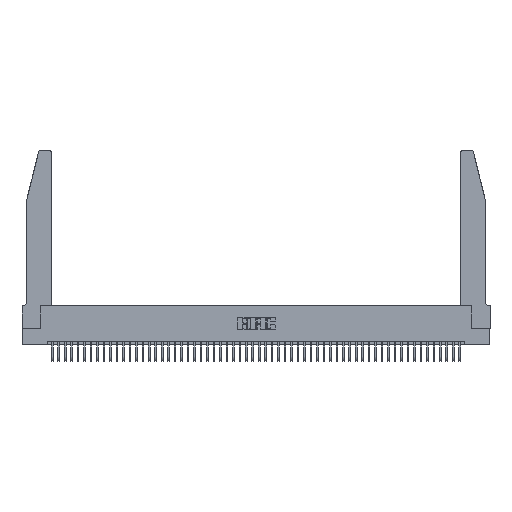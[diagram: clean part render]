
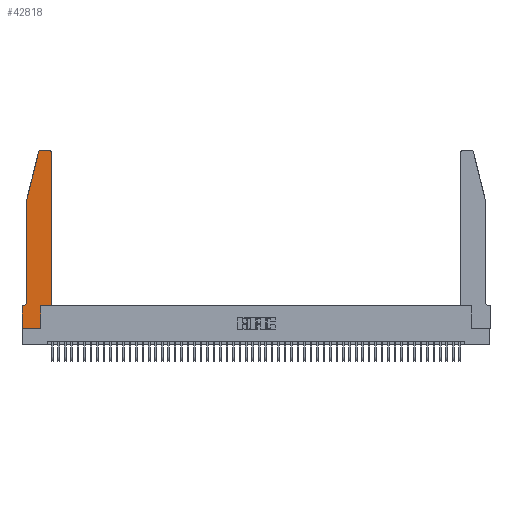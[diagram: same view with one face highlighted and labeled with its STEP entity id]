
A CAD part, top view. The second image highlights one B-rep face of the part: STEP entity #42818.
In plain terms, the highlighted planar face has unit normal (0, 0, 1).
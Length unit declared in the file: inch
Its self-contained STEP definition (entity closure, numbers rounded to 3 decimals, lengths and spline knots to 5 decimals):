
#432 = CARTESIAN_POINT ( 'NONE',  ( 0.4505, 0.35, 0.37 ) ) ;
#1032 = ORIENTED_EDGE ( 'NONE', *, *, #32963, .T. ) ;
#1326 = ORIENTED_EDGE ( 'NONE', *, *, #33201, .T. ) ;
#2645 = VERTEX_POINT ( 'NONE', #17183 ) ;
#3029 = EDGE_CURVE ( 'NONE', #3088, #14454, #19236, .T. ) ;
#3088 = VERTEX_POINT ( 'NONE', #35722 ) ;
#3173 = ORIENTED_EDGE ( 'NONE', *, *, #40153, .T. ) ;
#3395 = ORIENTED_EDGE ( 'NONE', *, *, #49207, .T. ) ;
#3697 = VERTEX_POINT ( 'NONE', #4847 ) ;
#4013 = VECTOR ( 'NONE', #29248, 39.37008 ) ;
#4138 = CARTESIAN_POINT ( 'NONE',  ( 0.4205, 2.75, 0.37 ) ) ;
#4597 = LINE ( 'NONE', #30398, #33091 ) ;
#4698 = VERTEX_POINT ( 'NONE', #19447 ) ;
#4748 = EDGE_CURVE ( 'NONE', #10122, #2645, #46123, .T. ) ;
#4847 = CARTESIAN_POINT ( 'NONE',  ( 0.0755, 2., 0.37 ) ) ;
#6041 = LINE ( 'NONE', #33193, #32089 ) ;
#6092 = DIRECTION ( 'NONE',  ( 0., -1., 0. ) ) ;
#6911 = PLANE ( 'NONE',  #46833 ) ;
#7537 = LINE ( 'NONE', #32663, #26944 ) ;
#7711 = VECTOR ( 'NONE', #12213, 39.37008 ) ;
#7830 = CARTESIAN_POINT ( 'NONE',  ( 0.2865, 0.35, 0.37 ) ) ;
#7932 = DIRECTION ( 'NONE',  ( 0., 1., 0. ) ) ;
#8380 = DIRECTION ( 'NONE',  ( 0., 0., 1. ) ) ;
#8432 = VERTEX_POINT ( 'NONE', #39535 ) ;
#8803 = DIRECTION ( 'NONE',  ( -1., 0., 0. ) ) ;
#9046 = VECTOR ( 'NONE', #46430, 39.37008 ) ;
#9170 = VERTEX_POINT ( 'NONE', #40303 ) ;
#9716 = CARTESIAN_POINT ( 'NONE',  ( 0.25487, 2.72718, 0.37 ) ) ;
#9871 = DIRECTION ( 'NONE',  ( 0., 0., 1. ) ) ;
#10122 = VERTEX_POINT ( 'NONE', #17266 ) ;
#10982 = DIRECTION ( 'NONE',  ( 1., 0., 0. ) ) ;
#11232 = VERTEX_POINT ( 'NONE', #23738 ) ;
#12045 = DIRECTION ( 'NONE',  ( -0.239, -0.971, 0. ) ) ;
#12158 = CIRCLE ( 'NONE', #20756, 0.03 ) ;
#12213 = DIRECTION ( 'NONE',  ( 1., 0., 0. ) ) ;
#14454 = VERTEX_POINT ( 'NONE', #16773 ) ;
#14485 = EDGE_CURVE ( 'NONE', #20137, #9170, #22535, .T. ) ;
#15558 = EDGE_CURVE ( 'NONE', #3697, #4698, #6041, .T. ) ;
#16773 = CARTESIAN_POINT ( 'NONE',  ( 0.2865, 0., 0.37 ) ) ;
#16843 = CARTESIAN_POINT ( 'NONE',  ( 0.0055, 0.42, 0.37 ) ) ;
#17183 = CARTESIAN_POINT ( 'NONE',  ( 0.4505, 2.72, 0.37 ) ) ;
#17266 = CARTESIAN_POINT ( 'NONE',  ( 0.4505, 0.35, 0.37 ) ) ;
#17850 = VECTOR ( 'NONE', #7932, 39.37008 ) ;
#19236 = LINE ( 'NONE', #46759, #7711 ) ;
#19326 = LINE ( 'NONE', #7830, #9046 ) ;
#19447 = CARTESIAN_POINT ( 'NONE',  ( 0.0755, 0.42, 0.37 ) ) ;
#19665 = CARTESIAN_POINT ( 'NONE',  ( 0.0755, 2., 0.37 ) ) ;
#19840 = ORIENTED_EDGE ( 'NONE', *, *, #4748, .T. ) ;
#20137 = VERTEX_POINT ( 'NONE', #28418 ) ;
#20263 = ORIENTED_EDGE ( 'NONE', *, *, #34216, .T. ) ;
#20718 = DIRECTION ( 'NONE',  ( -1., 0., 0. ) ) ;
#20756 = AXIS2_PLACEMENT_3D ( 'NONE', #31556, #8380, #35433 ) ;
#20955 = CIRCLE ( 'NONE', #39477, 0.07 ) ;
#21087 = ORIENTED_EDGE ( 'NONE', *, *, #3029, .T. ) ;
#21795 = VECTOR ( 'NONE', #12045, 39.37008 ) ;
#22535 = LINE ( 'NONE', #24539, #34027 ) ;
#23369 = EDGE_CURVE ( 'NONE', #8432, #48941, #49300, .T. ) ;
#23738 = CARTESIAN_POINT ( 'NONE',  ( 0.2865, 0.35, 0.37 ) ) ;
#24539 = CARTESIAN_POINT ( 'NONE',  ( 0.0755, 0.35, 0.37 ) ) ;
#26944 = VECTOR ( 'NONE', #32487, 39.37008 ) ;
#27886 = ORIENTED_EDGE ( 'NONE', *, *, #15558, .T. ) ;
#28418 = CARTESIAN_POINT ( 'NONE',  ( 0.0055, 0.35, 0.37 ) ) ;
#28450 = ORIENTED_EDGE ( 'NONE', *, *, #43547, .T. ) ;
#29248 = DIRECTION ( 'NONE',  ( 1., 0., 0. ) ) ;
#29536 = ORIENTED_EDGE ( 'NONE', *, *, #23369, .T. ) ;
#29956 = VERTEX_POINT ( 'NONE', #4138 ) ;
#30398 = CARTESIAN_POINT ( 'NONE',  ( 0.2605, 2.75, 0.37 ) ) ;
#31556 = CARTESIAN_POINT ( 'NONE',  ( 0.4205, 2.72, 0.37 ) ) ;
#32071 = LINE ( 'NONE', #19665, #21795 ) ;
#32089 = VECTOR ( 'NONE', #6092, 39.37008 ) ;
#32209 = FACE_OUTER_BOUND ( 'NONE', #48588, .T. ) ;
#32487 = DIRECTION ( 'NONE',  ( 0., -1., 0. ) ) ;
#32663 = CARTESIAN_POINT ( 'NONE',  ( 0., 0., 0.37 ) ) ;
#32963 = EDGE_CURVE ( 'NONE', #11232, #10122, #34915, .T. ) ;
#33033 = CARTESIAN_POINT ( 'NONE',  ( 0.284, 2.72, 0.37 ) ) ;
#33091 = VECTOR ( 'NONE', #49341, 39.37008 ) ;
#33193 = CARTESIAN_POINT ( 'NONE',  ( 0.0755, 2., 0.37 ) ) ;
#33201 = EDGE_CURVE ( 'NONE', #29956, #8432, #4597, .T. ) ;
#33517 = EDGE_CURVE ( 'NONE', #4698, #20137, #20955, .T. ) ;
#34027 = VECTOR ( 'NONE', #8803, 39.37008 ) ;
#34155 = DIRECTION ( 'NONE',  ( 0., 0., 1. ) ) ;
#34216 = EDGE_CURVE ( 'NONE', #9170, #3088, #7537, .T. ) ;
#34915 = LINE ( 'NONE', #48341, #4013 ) ;
#35433 = DIRECTION ( 'NONE',  ( 1., 0., 0. ) ) ;
#35722 = CARTESIAN_POINT ( 'NONE',  ( 0., 0., 0.37 ) ) ;
#36889 = DIRECTION ( 'NONE',  ( 1., 0., 0. ) ) ;
#39477 = AXIS2_PLACEMENT_3D ( 'NONE', #16843, #43776, #20718 ) ;
#39535 = CARTESIAN_POINT ( 'NONE',  ( 0.284, 2.75, 0.37 ) ) ;
#40153 = EDGE_CURVE ( 'NONE', #14454, #11232, #19326, .T. ) ;
#40303 = CARTESIAN_POINT ( 'NONE',  ( 0., 0.35, 0.37 ) ) ;
#41368 = ORIENTED_EDGE ( 'NONE', *, *, #33517, .T. ) ;
#42818 = ADVANCED_FACE ( 'NONE', ( #32209 ), #6911, .T. ) ;
#43547 = EDGE_CURVE ( 'NONE', #2645, #29956, #12158, .T. ) ;
#43776 = DIRECTION ( 'NONE',  ( 0., 0., -1. ) ) ;
#46123 = LINE ( 'NONE', #432, #17850 ) ;
#46430 = DIRECTION ( 'NONE',  ( 0., 1., 0. ) ) ;
#46759 = CARTESIAN_POINT ( 'NONE',  ( 0., 0., 0.37 ) ) ;
#46833 = AXIS2_PLACEMENT_3D ( 'NONE', #49393, #34155, #10982 ) ;
#47065 = AXIS2_PLACEMENT_3D ( 'NONE', #33033, #9871, #36889 ) ;
#48341 = CARTESIAN_POINT ( 'NONE',  ( 0.4505, 0.35, 0.37 ) ) ;
#48588 = EDGE_LOOP ( 'NONE', ( #1326, #29536, #3395, #27886, #41368, #49679, #20263, #21087, #3173, #1032, #19840, #28450 ) ) ;
#48941 = VERTEX_POINT ( 'NONE', #9716 ) ;
#49207 = EDGE_CURVE ( 'NONE', #48941, #3697, #32071, .T. ) ;
#49300 = CIRCLE ( 'NONE', #47065, 0.03 ) ;
#49341 = DIRECTION ( 'NONE',  ( -1., 0., 0. ) ) ;
#49393 = CARTESIAN_POINT ( 'NONE',  ( 0., 0.35, 0.37 ) ) ;
#49679 = ORIENTED_EDGE ( 'NONE', *, *, #14485, .T. ) ;
